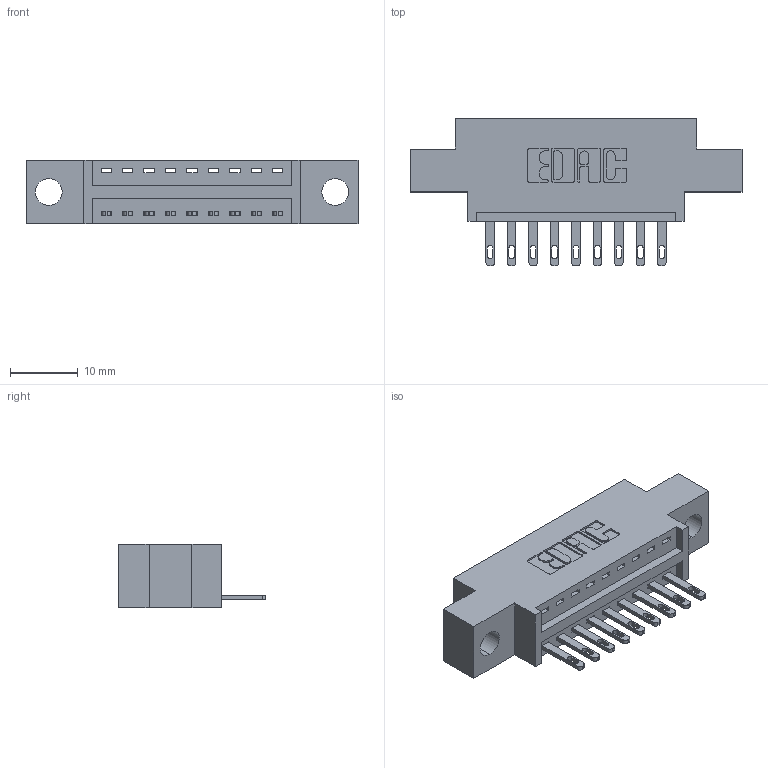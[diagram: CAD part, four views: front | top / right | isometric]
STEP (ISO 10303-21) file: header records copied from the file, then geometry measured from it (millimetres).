
FILE_DESCRIPTION (( 'STEP AP203' ), '1' );
FILE_NAME ('896-009-500-604.STEP', '2021-07-27T14:11:16', ( '' ), ( '' ), 'SwSTEP 2.0', 'SolidWorks 2020', '' );
FILE_SCHEMA (( 'CONFIG_CONTROL_DESIGN' ));
Length unit declared in the file: inch
Products named in the file (3): 846 Part_0.170 Offset - 0.156 Dia-TH; 896-009-500-604; 345-292-001_345-293-100
Assembly tree (10 placements, depth 2):
  896-009-500-604
    846 Part_0.170 Offset - 0.156 Dia-TH
    345-292-001_345-293-100  x9
Bounding box: 49.15 x 21.84 x 9.4 mm (x, y, z)
Volume: 4240.4 mm3; surface area: 4930.1 mm2
Topology: 10 solids, 10 shells, 612 faces, 1853 edges, 1234 vertices
Faces by surface type: plane 386, cylinder 226
Entity records: 10093 total; most frequent: CARTESIAN_POINT 1747, ORIENTED_EDGE 1690, DIRECTION 1583, EDGE_CURVE 845, LINE 673, VECTOR 673, VERTEX_POINT 562, AXIS2_PLACEMENT_3D 455
